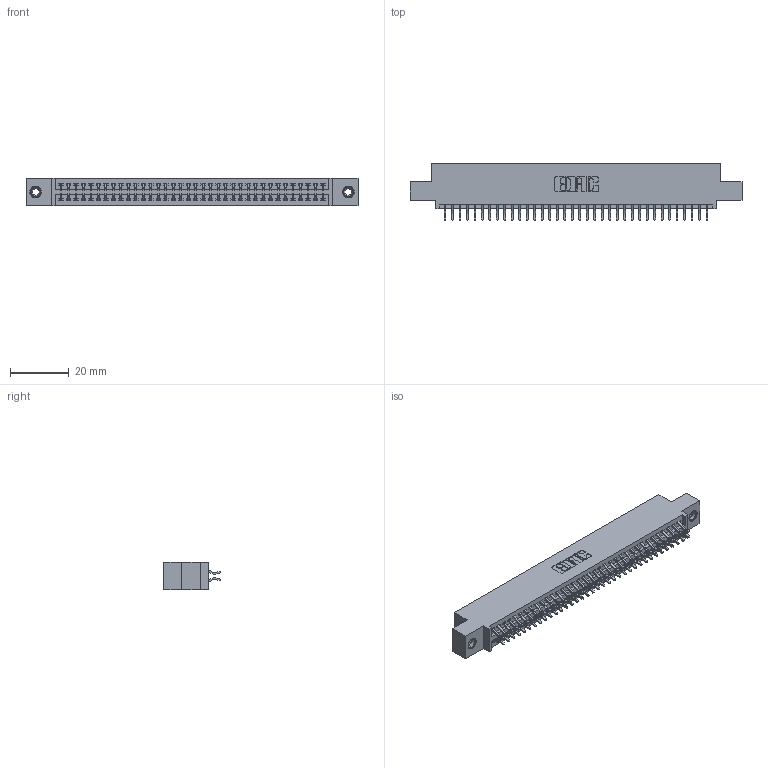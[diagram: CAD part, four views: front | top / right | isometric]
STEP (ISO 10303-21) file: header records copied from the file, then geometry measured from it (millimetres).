
FILE_DESCRIPTION (( 'STEP AP203' ), '1' );
FILE_NAME ('345-072-556-508.STEP', '2019-10-31T04:31:44', ( '' ), ( '' ), 'SwSTEP 2.0', 'SolidWorks 2016', '' );
FILE_SCHEMA (( 'CONFIG_CONTROL_DESIGN' ));
Length unit declared in the file: inch
Products named in the file (4): 345-250-001_345-250-003-102; 345 Part_0.110 Offset - 0.156 Dia-TI; 345-072-556-508; 345-292-001_556 Tail
Assembly tree (75 placements, depth 2):
  345-072-556-508
    345 Part_0.110 Offset - 0.156 Dia-TI
    345-292-001_556 Tail  x72
    345-250-001_345-250-003-102  x2
Bounding box: 112.65 x 19.24 x 9.4 mm (x, y, z)
Volume: 10804.4 mm3; surface area: 15897.8 mm2
Topology: 75 solids, 75 shells, 4222 faces, 12513 edges, 8238 vertices
Faces by surface type: plane 2780, cylinder 1426, cone 12, torus 4
Entity records: 30592 total; most frequent: CARTESIAN_POINT 5131, ORIENTED_EDGE 5046, DIRECTION 4545, EDGE_CURVE 2523, VECTOR 2219, LINE 2219, VERTEX_POINT 1676, AXIS2_PLACEMENT_3D 1163
